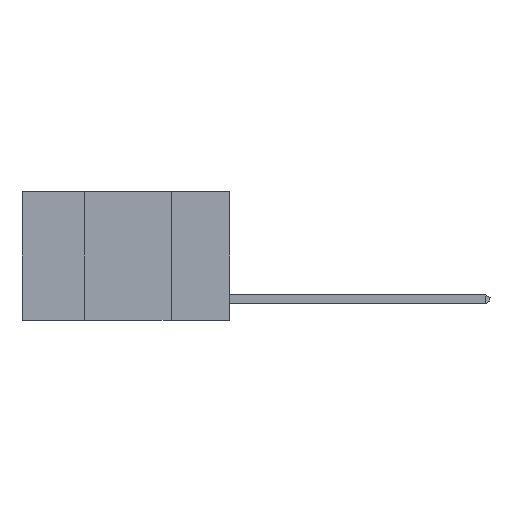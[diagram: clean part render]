
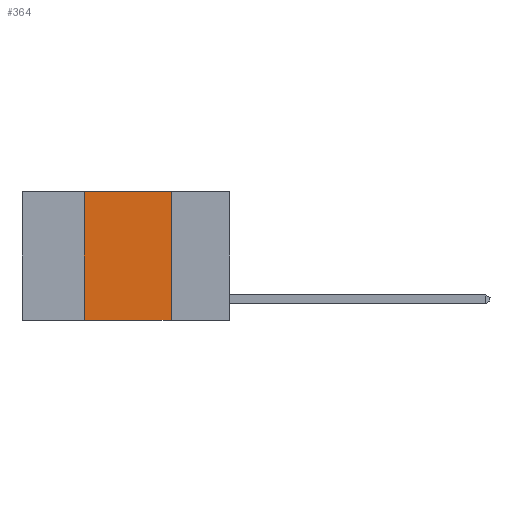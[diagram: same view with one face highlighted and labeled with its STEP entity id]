
A CAD part, left-side view. The second image highlights one B-rep face of the part: STEP entity #364.
In plain terms, the highlighted planar face has unit normal (-1, 0, 0).
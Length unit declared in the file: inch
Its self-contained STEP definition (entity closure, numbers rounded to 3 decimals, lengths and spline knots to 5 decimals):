
#146 = ORIENTED_EDGE ( 'NONE', *, *, #6625, .F. ) ;
#364 = ADVANCED_FACE ( 'NONE', ( #1106 ), #8919, .F. ) ;
#972 = LINE ( 'NONE', #21953, #16070 ) ;
#1106 = FACE_OUTER_BOUND ( 'NONE', #6455, .T. ) ;
#1800 = DIRECTION ( 'NONE',  ( 0., 0., 1. ) ) ;
#2222 = ORIENTED_EDGE ( 'NONE', *, *, #18749, .T. ) ;
#4303 = DIRECTION ( 'NONE',  ( 0., 0., -1. ) ) ;
#4356 = AXIS2_PLACEMENT_3D ( 'NONE', #16693, #20668, #18759 ) ;
#4670 = VECTOR ( 'NONE', #21715, 39.37008 ) ;
#5008 = CARTESIAN_POINT ( 'NONE',  ( 0., 0.42, 0. ) ) ;
#5430 = CARTESIAN_POINT ( 'NONE',  ( 0., 0.17, 0. ) ) ;
#6106 = VECTOR ( 'NONE', #1800, 39.37008 ) ;
#6140 = LINE ( 'NONE', #13915, #4670 ) ;
#6455 = EDGE_LOOP ( 'NONE', ( #14771, #146, #23243, #2222 ) ) ;
#6625 = EDGE_CURVE ( 'NONE', #13678, #15249, #6140, .T. ) ;
#8868 = LINE ( 'NONE', #5008, #6106 ) ;
#8919 = PLANE ( 'NONE',  #4356 ) ;
#9074 = VERTEX_POINT ( 'NONE', #13527 ) ;
#9540 = CARTESIAN_POINT ( 'NONE',  ( 0., 0.42, 0. ) ) ;
#9912 = LINE ( 'NONE', #16172, #18354 ) ;
#10000 = CARTESIAN_POINT ( 'NONE',  ( 0., 0.42, -0.37 ) ) ;
#10671 = DIRECTION ( 'NONE',  ( 0., -1., 0. ) ) ;
#13527 = CARTESIAN_POINT ( 'NONE',  ( 0., 0.17, -0.37 ) ) ;
#13678 = VERTEX_POINT ( 'NONE', #9540 ) ;
#13915 = CARTESIAN_POINT ( 'NONE',  ( 0., 0.6, 0. ) ) ;
#13920 = EDGE_CURVE ( 'NONE', #15249, #9074, #9912, .T. ) ;
#14771 = ORIENTED_EDGE ( 'NONE', *, *, #13920, .F. ) ;
#15249 = VERTEX_POINT ( 'NONE', #5430 ) ;
#15653 = EDGE_CURVE ( 'NONE', #21770, #13678, #8868, .T. ) ;
#16070 = VECTOR ( 'NONE', #10671, 39.37008 ) ;
#16172 = CARTESIAN_POINT ( 'NONE',  ( 0., 0.17, 0. ) ) ;
#16693 = CARTESIAN_POINT ( 'NONE',  ( 0., 0.6, 0. ) ) ;
#18354 = VECTOR ( 'NONE', #4303, 39.37008 ) ;
#18749 = EDGE_CURVE ( 'NONE', #21770, #9074, #972, .T. ) ;
#18759 = DIRECTION ( 'NONE',  ( 0., 0., -1. ) ) ;
#20668 = DIRECTION ( 'NONE',  ( 1., 0., 0. ) ) ;
#21715 = DIRECTION ( 'NONE',  ( 0., -1., 0. ) ) ;
#21770 = VERTEX_POINT ( 'NONE', #10000 ) ;
#21953 = CARTESIAN_POINT ( 'NONE',  ( 0., 0.6, -0.37 ) ) ;
#23243 = ORIENTED_EDGE ( 'NONE', *, *, #15653, .F. ) ;
